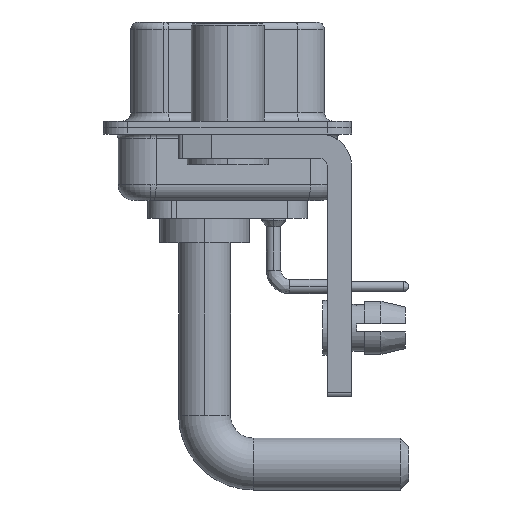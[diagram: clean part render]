
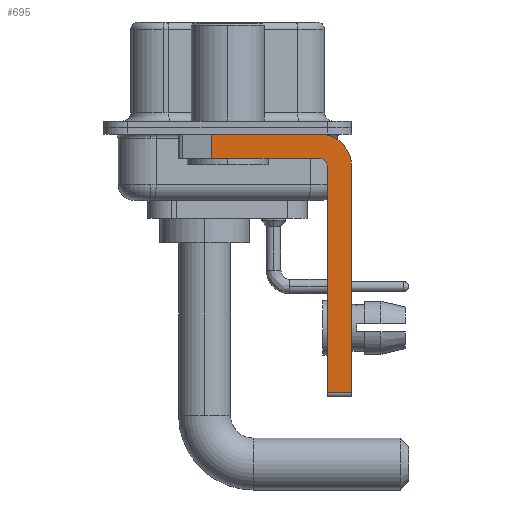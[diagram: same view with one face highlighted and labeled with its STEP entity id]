
A CAD part, left-side view. The second image highlights one B-rep face of the part: STEP entity #695.
In plain terms, the highlighted planar face has unit normal (-1, 0, 0).
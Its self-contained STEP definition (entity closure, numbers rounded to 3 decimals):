
#156 = VECTOR ( 'NONE', #15946, 1000. ) ;
#695 = ADVANCED_FACE ( 'NONE', ( #8580 ), #21047, .F. ) ;
#780 = VERTEX_POINT ( 'NONE', #11614 ) ;
#1170 = VERTEX_POINT ( 'NONE', #4517 ) ;
#1487 = ORIENTED_EDGE ( 'NONE', *, *, #10513, .F. ) ;
#1851 = VECTOR ( 'NONE', #18570, 1000. ) ;
#2523 = DIRECTION ( 'NONE',  ( 0., 1., 0. ) ) ;
#2701 = CARTESIAN_POINT ( 'NONE',  ( -2.9, 0.978, -1.9 ) ) ;
#3217 = DIRECTION ( 'NONE',  ( 0., 0., -1. ) ) ;
#3342 = VERTEX_POINT ( 'NONE', #10039 ) ;
#3478 = CARTESIAN_POINT ( 'NONE',  ( -2.9, 3., -0.4 ) ) ;
#4517 = CARTESIAN_POINT ( 'NONE',  ( -2.9, -7.65, -16.35 ) ) ;
#4999 = EDGE_CURVE ( 'NONE', #780, #10399, #25541, .T. ) ;
#5063 = DIRECTION ( 'NONE',  ( 0., -1., 0. ) ) ;
#5162 = VERTEX_POINT ( 'NONE', #19839 ) ;
#5618 = EDGE_LOOP ( 'NONE', ( #1487, #7092, #21504, #12065, #22294, #10163, #7100, #22341 ) ) ;
#6027 = AXIS2_PLACEMENT_3D ( 'NONE', #6908, #23542, #23675 ) ;
#6561 = CARTESIAN_POINT ( 'NONE',  ( -2.9, 0.978, -1.9 ) ) ;
#6908 = CARTESIAN_POINT ( 'NONE',  ( -2.9, -5.65, -2.4 ) ) ;
#7092 = ORIENTED_EDGE ( 'NONE', *, *, #20165, .T. ) ;
#7100 = ORIENTED_EDGE ( 'NONE', *, *, #21527, .F. ) ;
#7141 = LINE ( 'NONE', #19740, #12360 ) ;
#7589 = VECTOR ( 'NONE', #23307, 1000. ) ;
#7893 = EDGE_CURVE ( 'NONE', #3342, #1170, #7141, .T. ) ;
#8478 = EDGE_CURVE ( 'NONE', #5162, #12162, #12816, .T. ) ;
#8580 = FACE_OUTER_BOUND ( 'NONE', #5618, .T. ) ;
#8705 = AXIS2_PLACEMENT_3D ( 'NONE', #19685, #9582, #24243 ) ;
#9232 = VECTOR ( 'NONE', #2523, 1000. ) ;
#9472 = DIRECTION ( 'NONE',  ( 1., 0., 0. ) ) ;
#9582 = DIRECTION ( 'NONE',  ( -1., 0., 0. ) ) ;
#10039 = CARTESIAN_POINT ( 'NONE',  ( -2.9, -6.15, -16.35 ) ) ;
#10163 = ORIENTED_EDGE ( 'NONE', *, *, #7893, .T. ) ;
#10399 = VERTEX_POINT ( 'NONE', #2701 ) ;
#10513 = EDGE_CURVE ( 'NONE', #17508, #5162, #12215, .T. ) ;
#11463 = CARTESIAN_POINT ( 'NONE',  ( -2.9, -6.15, -2.4 ) ) ;
#11614 = CARTESIAN_POINT ( 'NONE',  ( -2.9, -5.65, -1.9 ) ) ;
#12065 = ORIENTED_EDGE ( 'NONE', *, *, #24740, .F. ) ;
#12162 = VERTEX_POINT ( 'NONE', #26054 ) ;
#12215 = LINE ( 'NONE', #3478, #1851 ) ;
#12360 = VECTOR ( 'NONE', #5063, 1000. ) ;
#12816 = CIRCLE ( 'NONE', #15903, 2. ) ;
#14578 = LINE ( 'NONE', #23035, #7589 ) ;
#15673 = LINE ( 'NONE', #26359, #27152 ) ;
#15903 = AXIS2_PLACEMENT_3D ( 'NONE', #24133, #9472, #26642 ) ;
#15946 = DIRECTION ( 'NONE',  ( 0., 0., -1. ) ) ;
#17088 = CIRCLE ( 'NONE', #8705, 0.5 ) ;
#17508 = VERTEX_POINT ( 'NONE', #19009 ) ;
#17621 = EDGE_CURVE ( 'NONE', #3342, #22416, #14578, .T. ) ;
#18570 = DIRECTION ( 'NONE',  ( 0., -1., 0. ) ) ;
#19009 = CARTESIAN_POINT ( 'NONE',  ( -2.9, 0.978, -0.4 ) ) ;
#19685 = CARTESIAN_POINT ( 'NONE',  ( -2.9, -5.65, -2.4 ) ) ;
#19740 = CARTESIAN_POINT ( 'NONE',  ( -2.9, -5.65, -16.35 ) ) ;
#19839 = CARTESIAN_POINT ( 'NONE',  ( -2.9, -5.65, -0.4 ) ) ;
#20165 = EDGE_CURVE ( 'NONE', #17508, #10399, #25543, .T. ) ;
#21047 = PLANE ( 'NONE',  #6027 ) ;
#21100 = CARTESIAN_POINT ( 'NONE',  ( -2.9, -5.65, -1.9 ) ) ;
#21504 = ORIENTED_EDGE ( 'NONE', *, *, #4999, .F. ) ;
#21527 = EDGE_CURVE ( 'NONE', #12162, #1170, #15673, .T. ) ;
#22294 = ORIENTED_EDGE ( 'NONE', *, *, #17621, .F. ) ;
#22341 = ORIENTED_EDGE ( 'NONE', *, *, #8478, .F. ) ;
#22416 = VERTEX_POINT ( 'NONE', #11463 ) ;
#23035 = CARTESIAN_POINT ( 'NONE',  ( -2.9, -6.15, -16.6 ) ) ;
#23307 = DIRECTION ( 'NONE',  ( 0., 0., 1. ) ) ;
#23542 = DIRECTION ( 'NONE',  ( 1., 0., 0. ) ) ;
#23675 = DIRECTION ( 'NONE',  ( 0., 0., -1. ) ) ;
#24133 = CARTESIAN_POINT ( 'NONE',  ( -2.9, -5.65, -2.4 ) ) ;
#24243 = DIRECTION ( 'NONE',  ( 0., 0., 1. ) ) ;
#24740 = EDGE_CURVE ( 'NONE', #22416, #780, #17088, .T. ) ;
#25541 = LINE ( 'NONE', #21100, #9232 ) ;
#25543 = LINE ( 'NONE', #6561, #156 ) ;
#26054 = CARTESIAN_POINT ( 'NONE',  ( -2.9, -7.65, -2.4 ) ) ;
#26359 = CARTESIAN_POINT ( 'NONE',  ( -2.9, -7.65, -2.4 ) ) ;
#26642 = DIRECTION ( 'NONE',  ( 0., 0., -1. ) ) ;
#27152 = VECTOR ( 'NONE', #3217, 1000. ) ;
